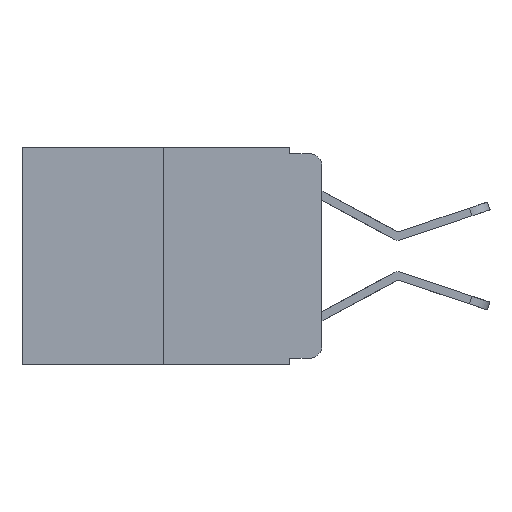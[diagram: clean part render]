
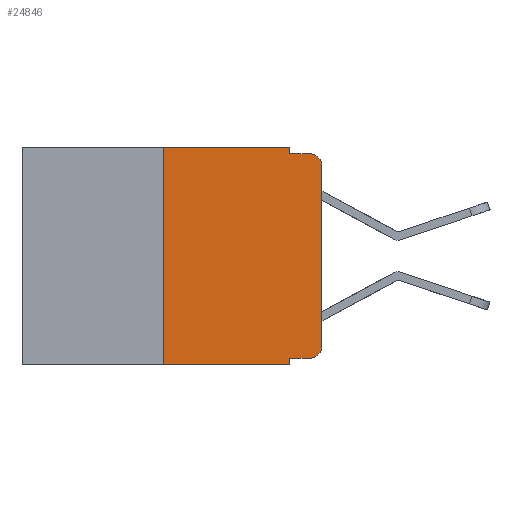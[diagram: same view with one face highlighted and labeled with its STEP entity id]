
A CAD part, left-side view. The second image highlights one B-rep face of the part: STEP entity #24846.
In plain terms, the highlighted planar face has unit normal (-1, 0, 0).
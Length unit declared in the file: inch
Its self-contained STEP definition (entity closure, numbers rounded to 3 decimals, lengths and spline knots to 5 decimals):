
#128 = CARTESIAN_POINT ( 'NONE',  ( 0., 0.051, 0. ) ) ;
#231 = EDGE_CURVE ( 'NONE', #16344, #17459, #24617, .T. ) ;
#308 = PLANE ( 'NONE',  #15961 ) ;
#443 = ORIENTED_EDGE ( 'NONE', *, *, #11903, .T. ) ;
#454 = CARTESIAN_POINT ( 'NONE',  ( 0., 0.051, 0. ) ) ;
#588 = CARTESIAN_POINT ( 'NONE',  ( 0., 0.051, -0.01 ) ) ;
#715 = VERTEX_POINT ( 'NONE', #12258 ) ;
#1064 = ORIENTED_EDGE ( 'NONE', *, *, #6783, .T. ) ;
#1117 = ORIENTED_EDGE ( 'NONE', *, *, #15683, .F. ) ;
#1862 = ORIENTED_EDGE ( 'NONE', *, *, #3914, .F. ) ;
#2348 = DIRECTION ( 'NONE',  ( 0., 0., -1. ) ) ;
#2529 = ORIENTED_EDGE ( 'NONE', *, *, #11869, .F. ) ;
#2632 = VECTOR ( 'NONE', #22905, 39.37008 ) ;
#2740 = CARTESIAN_POINT ( 'NONE',  ( 0., 0.051, -0.343 ) ) ;
#2827 = ORIENTED_EDGE ( 'NONE', *, *, #12929, .F. ) ;
#3316 = LINE ( 'NONE', #6507, #2632 ) ;
#3578 = LINE ( 'NONE', #22140, #24202 ) ;
#3610 = ORIENTED_EDGE ( 'NONE', *, *, #231, .T. ) ;
#3858 = ORIENTED_EDGE ( 'NONE', *, *, #8213, .F. ) ;
#3914 = EDGE_CURVE ( 'NONE', #4765, #4104, #17912, .T. ) ;
#4075 = LINE ( 'NONE', #128, #25279 ) ;
#4104 = VERTEX_POINT ( 'NONE', #588 ) ;
#4126 = DIRECTION ( 'NONE',  ( -1., 0., 0. ) ) ;
#4136 = CARTESIAN_POINT ( 'NONE',  ( 0., 0.02, -0.313 ) ) ;
#4279 = ORIENTED_EDGE ( 'NONE', *, *, #11029, .T. ) ;
#4458 = DIRECTION ( 'NONE',  ( 0., -1., 0. ) ) ;
#4474 = ORIENTED_EDGE ( 'NONE', *, *, #12419, .T. ) ;
#4499 = DIRECTION ( 'NONE',  ( 0., -1., 0. ) ) ;
#4765 = VERTEX_POINT ( 'NONE', #454 ) ;
#5565 = VECTOR ( 'NONE', #20756, 39.37008 ) ;
#6297 = DIRECTION ( 'NONE',  ( 0., 0., -1. ) ) ;
#6507 = CARTESIAN_POINT ( 'NONE',  ( 0., 0.473, 0. ) ) ;
#6783 = EDGE_CURVE ( 'NONE', #715, #26210, #10486, .T. ) ;
#7578 = DIRECTION ( 'NONE',  ( 0., -1., 0. ) ) ;
#7743 = EDGE_LOOP ( 'NONE', ( #443, #1064, #1117, #1862, #2529, #2827, #3610, #3858, #4279, #4474 ) ) ;
#8213 = EDGE_CURVE ( 'NONE', #18820, #17459, #4075, .T. ) ;
#8439 = LINE ( 'NONE', #19878, #19997 ) ;
#8505 = CARTESIAN_POINT ( 'NONE',  ( 0., 0.051, 0. ) ) ;
#10486 = CIRCLE ( 'NONE', #13753, 0.02 ) ;
#10514 = CARTESIAN_POINT ( 'NONE',  ( 0., 0.02, -0.01 ) ) ;
#10623 = CIRCLE ( 'NONE', #16933, 0.02 ) ;
#10758 = CARTESIAN_POINT ( 'NONE',  ( 0., 0., 0. ) ) ;
#11029 = EDGE_CURVE ( 'NONE', #18820, #11443, #23379, .T. ) ;
#11443 = VERTEX_POINT ( 'NONE', #24584 ) ;
#11698 = CARTESIAN_POINT ( 'NONE',  ( 0., 0.051, -0.333 ) ) ;
#11869 = EDGE_CURVE ( 'NONE', #11899, #4765, #3316, .T. ) ;
#11899 = VERTEX_POINT ( 'NONE', #22989 ) ;
#11903 = EDGE_CURVE ( 'NONE', #15343, #715, #18006, .T. ) ;
#12258 = CARTESIAN_POINT ( 'NONE',  ( 0., 0., -0.03 ) ) ;
#12419 = EDGE_CURVE ( 'NONE', #11443, #15343, #10623, .T. ) ;
#12586 = VECTOR ( 'NONE', #24998, 39.37008 ) ;
#12929 = EDGE_CURVE ( 'NONE', #16344, #11899, #3578, .T. ) ;
#13159 = DIRECTION ( 'NONE',  ( 0., 0., -1. ) ) ;
#13753 = AXIS2_PLACEMENT_3D ( 'NONE', #16649, #4126, #18670 ) ;
#13904 = VECTOR ( 'NONE', #4458, 39.37008 ) ;
#15120 = CARTESIAN_POINT ( 'NONE',  ( 0., 0.473, 0. ) ) ;
#15343 = VERTEX_POINT ( 'NONE', #20847 ) ;
#15683 = EDGE_CURVE ( 'NONE', #4104, #26210, #8439, .T. ) ;
#15961 = AXIS2_PLACEMENT_3D ( 'NONE', #15120, #25226, #13159 ) ;
#16344 = VERTEX_POINT ( 'NONE', #17990 ) ;
#16649 = CARTESIAN_POINT ( 'NONE',  ( 0., 0.02, -0.03 ) ) ;
#16933 = AXIS2_PLACEMENT_3D ( 'NONE', #4136, #18673, #6297 ) ;
#17459 = VERTEX_POINT ( 'NONE', #2740 ) ;
#17912 = LINE ( 'NONE', #8505, #5565 ) ;
#17990 = CARTESIAN_POINT ( 'NONE',  ( 0., 0.25, -0.343 ) ) ;
#18006 = LINE ( 'NONE', #10758, #12586 ) ;
#18670 = DIRECTION ( 'NONE',  ( 0., 0., -1. ) ) ;
#18673 = DIRECTION ( 'NONE',  ( -1., 0., 0. ) ) ;
#18820 = VERTEX_POINT ( 'NONE', #11698 ) ;
#18916 = CARTESIAN_POINT ( 'NONE',  ( 0., 0.051, -0.333 ) ) ;
#18957 = CARTESIAN_POINT ( 'NONE',  ( 0., 0.473, -0.343 ) ) ;
#19878 = CARTESIAN_POINT ( 'NONE',  ( 0., 0.051, -0.01 ) ) ;
#19997 = VECTOR ( 'NONE', #7578, 39.37008 ) ;
#20756 = DIRECTION ( 'NONE',  ( 0., 0., -1. ) ) ;
#20847 = CARTESIAN_POINT ( 'NONE',  ( 0., 0., -0.313 ) ) ;
#21192 = FACE_OUTER_BOUND ( 'NONE', #7743, .T. ) ;
#22140 = CARTESIAN_POINT ( 'NONE',  ( 0., 0.25, 0. ) ) ;
#22759 = VECTOR ( 'NONE', #4499, 39.37008 ) ;
#22905 = DIRECTION ( 'NONE',  ( 0., -1., 0. ) ) ;
#22989 = CARTESIAN_POINT ( 'NONE',  ( 0., 0.25, 0. ) ) ;
#23379 = LINE ( 'NONE', #18916, #22759 ) ;
#24159 = DIRECTION ( 'NONE',  ( 0., 0., 1. ) ) ;
#24202 = VECTOR ( 'NONE', #24159, 39.37008 ) ;
#24584 = CARTESIAN_POINT ( 'NONE',  ( 0., 0.02, -0.333 ) ) ;
#24617 = LINE ( 'NONE', #18957, #13904 ) ;
#24846 = ADVANCED_FACE ( 'NONE', ( #21192 ), #308, .F. ) ;
#24998 = DIRECTION ( 'NONE',  ( 0., 0., 1. ) ) ;
#25226 = DIRECTION ( 'NONE',  ( 1., 0., 0. ) ) ;
#25279 = VECTOR ( 'NONE', #2348, 39.37008 ) ;
#26210 = VERTEX_POINT ( 'NONE', #10514 ) ;
